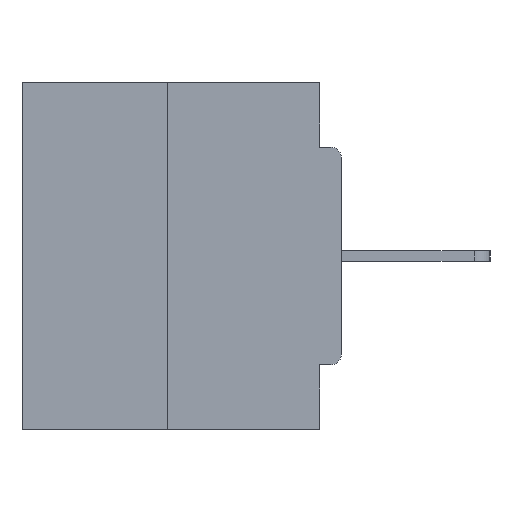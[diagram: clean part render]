
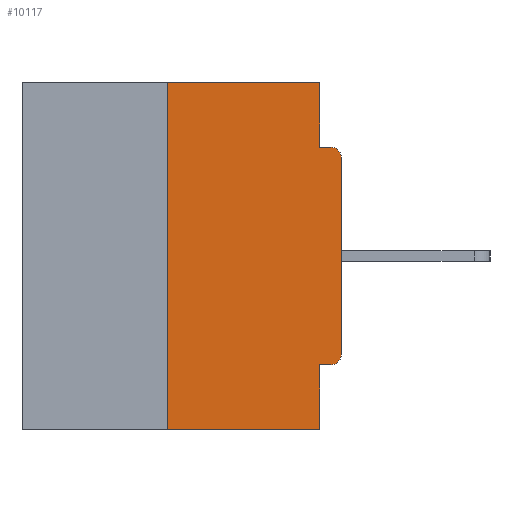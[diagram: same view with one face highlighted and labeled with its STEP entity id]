
A CAD part, left-side view. The second image highlights one B-rep face of the part: STEP entity #10117.
In plain terms, the highlighted planar face has unit normal (-1, 0, 0).
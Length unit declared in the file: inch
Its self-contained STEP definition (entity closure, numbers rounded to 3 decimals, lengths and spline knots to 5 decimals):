
#93 = VERTEX_POINT ( 'NONE', #18500 ) ;
#357 = ORIENTED_EDGE ( 'NONE', *, *, #21517, .F. ) ;
#618 = VERTEX_POINT ( 'NONE', #9945 ) ;
#686 = CARTESIAN_POINT ( 'NONE',  ( 0., 0., -0.3915 ) ) ;
#1900 = AXIS2_PLACEMENT_3D ( 'NONE', #30720, #25162, #3420 ) ;
#2093 = DIRECTION ( 'NONE',  ( 0., 0., -1. ) ) ;
#3001 = DIRECTION ( 'NONE',  ( 0., -1., 0. ) ) ;
#3093 = CARTESIAN_POINT ( 'NONE',  ( 0., 0.25, 0. ) ) ;
#3420 = DIRECTION ( 'NONE',  ( 0., 0., -1. ) ) ;
#3722 = CARTESIAN_POINT ( 'NONE',  ( 0., 0.015, -0.0935 ) ) ;
#4589 = VECTOR ( 'NONE', #18157, 39.37008 ) ;
#5113 = VERTEX_POINT ( 'NONE', #686 ) ;
#5518 = CARTESIAN_POINT ( 'NONE',  ( 0., 0.031, -0.5 ) ) ;
#6257 = ORIENTED_EDGE ( 'NONE', *, *, #15444, .T. ) ;
#6777 = CIRCLE ( 'NONE', #20338, 0.015 ) ;
#6920 = CARTESIAN_POINT ( 'NONE',  ( 0., 0.46, 0. ) ) ;
#7429 = CARTESIAN_POINT ( 'NONE',  ( 0., 0.031, -0.5 ) ) ;
#7623 = LINE ( 'NONE', #5518, #29784 ) ;
#8121 = LINE ( 'NONE', #13505, #11994 ) ;
#8200 = CARTESIAN_POINT ( 'NONE',  ( 0., 0., -0.0935 ) ) ;
#8281 = DIRECTION ( 'NONE',  ( 0., 1., 0. ) ) ;
#8310 = PLANE ( 'NONE',  #1900 ) ;
#8453 = ORIENTED_EDGE ( 'NONE', *, *, #11600, .F. ) ;
#8663 = LINE ( 'NONE', #18464, #16568 ) ;
#9277 = EDGE_LOOP ( 'NONE', ( #14630, #17560, #19946, #357, #20242, #20872, #6257, #15740, #8453, #30030 ) ) ;
#9435 = CARTESIAN_POINT ( 'NONE',  ( 0., 0.015, -0.1085 ) ) ;
#9454 = VERTEX_POINT ( 'NONE', #18545 ) ;
#9945 = CARTESIAN_POINT ( 'NONE',  ( 0., 0.015, -0.4065 ) ) ;
#10117 = ADVANCED_FACE ( 'NONE', ( #13373 ), #8310, .F. ) ;
#10431 = DIRECTION ( 'NONE',  ( 0., 0., 1. ) ) ;
#11287 = LINE ( 'NONE', #8200, #4589 ) ;
#11553 = VECTOR ( 'NONE', #8281, 39.37008 ) ;
#11599 = CARTESIAN_POINT ( 'NONE',  ( 0., 0.031, -0.0935 ) ) ;
#11600 = EDGE_CURVE ( 'NONE', #13425, #28893, #11287, .T. ) ;
#11994 = VECTOR ( 'NONE', #21021, 39.37008 ) ;
#13040 = LINE ( 'NONE', #3093, #20877 ) ;
#13373 = FACE_OUTER_BOUND ( 'NONE', #9277, .T. ) ;
#13425 = VERTEX_POINT ( 'NONE', #11599 ) ;
#13505 = CARTESIAN_POINT ( 'NONE',  ( 0., 0., 0. ) ) ;
#14508 = CARTESIAN_POINT ( 'NONE',  ( 0., 0.015, -0.3915 ) ) ;
#14630 = ORIENTED_EDGE ( 'NONE', *, *, #16184, .F. ) ;
#15179 = EDGE_CURVE ( 'NONE', #31899, #28893, #6777, .T. ) ;
#15444 = EDGE_CURVE ( 'NONE', #5113, #31899, #8121, .T. ) ;
#15740 = ORIENTED_EDGE ( 'NONE', *, *, #15179, .T. ) ;
#16184 = EDGE_CURVE ( 'NONE', #24527, #9454, #22611, .T. ) ;
#16310 = EDGE_CURVE ( 'NONE', #93, #30282, #20460, .T. ) ;
#16568 = VECTOR ( 'NONE', #21082, 39.37008 ) ;
#17378 = EDGE_CURVE ( 'NONE', #9454, #13425, #8663, .T. ) ;
#17560 = ORIENTED_EDGE ( 'NONE', *, *, #19576, .F. ) ;
#17812 = AXIS2_PLACEMENT_3D ( 'NONE', #14508, #24496, #2093 ) ;
#18157 = DIRECTION ( 'NONE',  ( 0., -1., 0. ) ) ;
#18242 = CARTESIAN_POINT ( 'NONE',  ( 0., 0., -0.4065 ) ) ;
#18464 = CARTESIAN_POINT ( 'NONE',  ( 0., 0.031, 0. ) ) ;
#18500 = CARTESIAN_POINT ( 'NONE',  ( 0., 0.25, -0.5 ) ) ;
#18545 = CARTESIAN_POINT ( 'NONE',  ( 0., 0.031, 0. ) ) ;
#19576 = EDGE_CURVE ( 'NONE', #93, #24527, #13040, .T. ) ;
#19693 = CARTESIAN_POINT ( 'NONE',  ( 0., 0.031, -0.4065 ) ) ;
#19946 = ORIENTED_EDGE ( 'NONE', *, *, #16310, .T. ) ;
#20242 = ORIENTED_EDGE ( 'NONE', *, *, #22836, .F. ) ;
#20338 = AXIS2_PLACEMENT_3D ( 'NONE', #9435, #24497, #29406 ) ;
#20460 = LINE ( 'NONE', #30457, #22291 ) ;
#20872 = ORIENTED_EDGE ( 'NONE', *, *, #22666, .T. ) ;
#20877 = VECTOR ( 'NONE', #10431, 39.37008 ) ;
#21021 = DIRECTION ( 'NONE',  ( 0., 0., 1. ) ) ;
#21082 = DIRECTION ( 'NONE',  ( 0., 0., -1. ) ) ;
#21492 = VECTOR ( 'NONE', #26878, 39.37008 ) ;
#21517 = EDGE_CURVE ( 'NONE', #30365, #30282, #7623, .T. ) ;
#22192 = DIRECTION ( 'NONE',  ( 0., 0., -1. ) ) ;
#22291 = VECTOR ( 'NONE', #3001, 39.37008 ) ;
#22611 = LINE ( 'NONE', #6920, #21492 ) ;
#22666 = EDGE_CURVE ( 'NONE', #618, #5113, #24101, .T. ) ;
#22836 = EDGE_CURVE ( 'NONE', #618, #30365, #23164, .T. ) ;
#23010 = CARTESIAN_POINT ( 'NONE',  ( 0., 0., -0.1085 ) ) ;
#23164 = LINE ( 'NONE', #18242, #11553 ) ;
#24101 = CIRCLE ( 'NONE', #17812, 0.015 ) ;
#24496 = DIRECTION ( 'NONE',  ( -1., 0., 0. ) ) ;
#24497 = DIRECTION ( 'NONE',  ( -1., 0., 0. ) ) ;
#24527 = VERTEX_POINT ( 'NONE', #28365 ) ;
#25162 = DIRECTION ( 'NONE',  ( 1., 0., 0. ) ) ;
#26878 = DIRECTION ( 'NONE',  ( 0., -1., 0. ) ) ;
#28365 = CARTESIAN_POINT ( 'NONE',  ( 0., 0.25, 0. ) ) ;
#28893 = VERTEX_POINT ( 'NONE', #3722 ) ;
#29406 = DIRECTION ( 'NONE',  ( 0., 0., -1. ) ) ;
#29784 = VECTOR ( 'NONE', #22192, 39.37008 ) ;
#30030 = ORIENTED_EDGE ( 'NONE', *, *, #17378, .F. ) ;
#30282 = VERTEX_POINT ( 'NONE', #7429 ) ;
#30365 = VERTEX_POINT ( 'NONE', #19693 ) ;
#30457 = CARTESIAN_POINT ( 'NONE',  ( 0., 0.46, -0.5 ) ) ;
#30720 = CARTESIAN_POINT ( 'NONE',  ( 0., 0.46, 0. ) ) ;
#31899 = VERTEX_POINT ( 'NONE', #23010 ) ;
